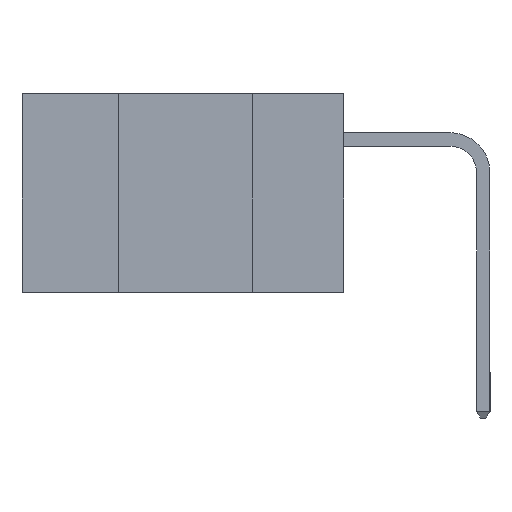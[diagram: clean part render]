
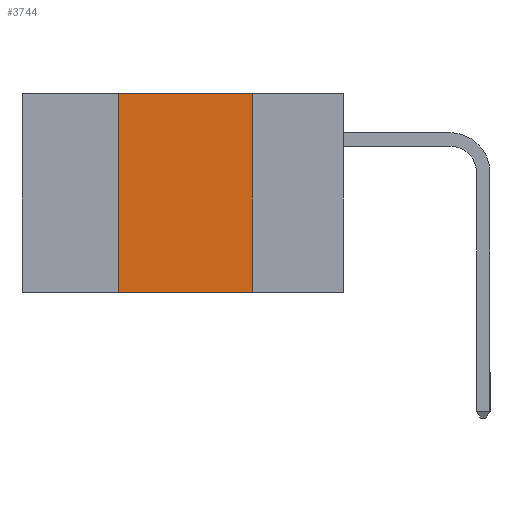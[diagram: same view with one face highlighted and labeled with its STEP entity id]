
A CAD part, left-side view. The second image highlights one B-rep face of the part: STEP entity #3744.
In plain terms, the highlighted planar face has unit normal (-1, 0, 0).
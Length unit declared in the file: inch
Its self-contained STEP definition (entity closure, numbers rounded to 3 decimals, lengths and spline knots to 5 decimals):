
#9 = DIRECTION ( 'NONE',  ( 0., -1., 0. ) ) ;
#793 = EDGE_CURVE ( 'NONE', #7316, #6249, #6687, .T. ) ;
#980 = ORIENTED_EDGE ( 'NONE', *, *, #793, .F. ) ;
#1559 = AXIS2_PLACEMENT_3D ( 'NONE', #7545, #5843, #4991 ) ;
#1864 = EDGE_LOOP ( 'NONE', ( #3857, #980, #7601, #8857 ) ) ;
#2590 = CARTESIAN_POINT ( 'NONE',  ( 0., 0.6, 0. ) ) ;
#2594 = CARTESIAN_POINT ( 'NONE',  ( 0., 0.42, -0.37 ) ) ;
#2804 = DIRECTION ( 'NONE',  ( 0., 0., -1. ) ) ;
#3042 = CARTESIAN_POINT ( 'NONE',  ( 0., 0.42, -0.37 ) ) ;
#3099 = VECTOR ( 'NONE', #2804, 39.37008 ) ;
#3262 = EDGE_CURVE ( 'NONE', #3749, #9584, #4051, .T. ) ;
#3736 = DIRECTION ( 'NONE',  ( 0., 0., 1. ) ) ;
#3744 = ADVANCED_FACE ( 'NONE', ( #7392 ), #4090, .F. ) ;
#3749 = VERTEX_POINT ( 'NONE', #2594 ) ;
#3857 = ORIENTED_EDGE ( 'NONE', *, *, #6573, .F. ) ;
#4051 = LINE ( 'NONE', #7296, #4942 ) ;
#4090 = PLANE ( 'NONE',  #1559 ) ;
#4942 = VECTOR ( 'NONE', #9, 39.37008 ) ;
#4991 = DIRECTION ( 'NONE',  ( 0., 0., -1. ) ) ;
#5376 = CARTESIAN_POINT ( 'NONE',  ( 0., 0.42, 0. ) ) ;
#5549 = LINE ( 'NONE', #3042, #6847 ) ;
#5843 = DIRECTION ( 'NONE',  ( 1., 0., 0. ) ) ;
#6099 = CARTESIAN_POINT ( 'NONE',  ( 0., 0.17, -0.37 ) ) ;
#6249 = VERTEX_POINT ( 'NONE', #7496 ) ;
#6573 = EDGE_CURVE ( 'NONE', #6249, #9584, #10006, .T. ) ;
#6687 = LINE ( 'NONE', #2590, #8639 ) ;
#6847 = VECTOR ( 'NONE', #3736, 39.37008 ) ;
#6990 = EDGE_CURVE ( 'NONE', #3749, #7316, #5549, .T. ) ;
#7296 = CARTESIAN_POINT ( 'NONE',  ( 0., 0.6, -0.37 ) ) ;
#7316 = VERTEX_POINT ( 'NONE', #5376 ) ;
#7392 = FACE_OUTER_BOUND ( 'NONE', #1864, .T. ) ;
#7496 = CARTESIAN_POINT ( 'NONE',  ( 0., 0.17, 0. ) ) ;
#7545 = CARTESIAN_POINT ( 'NONE',  ( 0., 0.6, 0. ) ) ;
#7601 = ORIENTED_EDGE ( 'NONE', *, *, #6990, .F. ) ;
#8639 = VECTOR ( 'NONE', #9070, 39.37008 ) ;
#8857 = ORIENTED_EDGE ( 'NONE', *, *, #3262, .T. ) ;
#9070 = DIRECTION ( 'NONE',  ( 0., -1., 0. ) ) ;
#9222 = CARTESIAN_POINT ( 'NONE',  ( 0., 0.17, -0.37 ) ) ;
#9584 = VERTEX_POINT ( 'NONE', #6099 ) ;
#10006 = LINE ( 'NONE', #9222, #3099 ) ;
